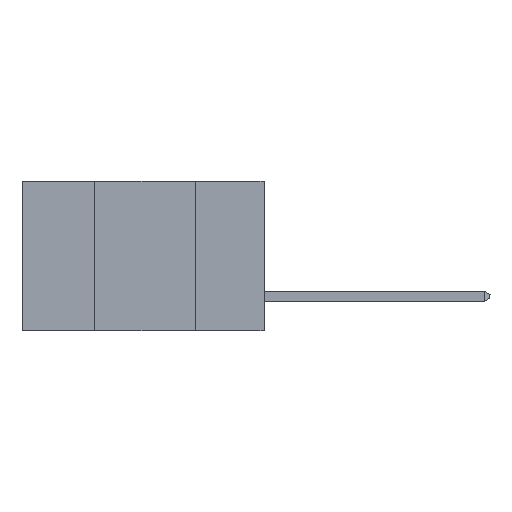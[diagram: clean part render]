
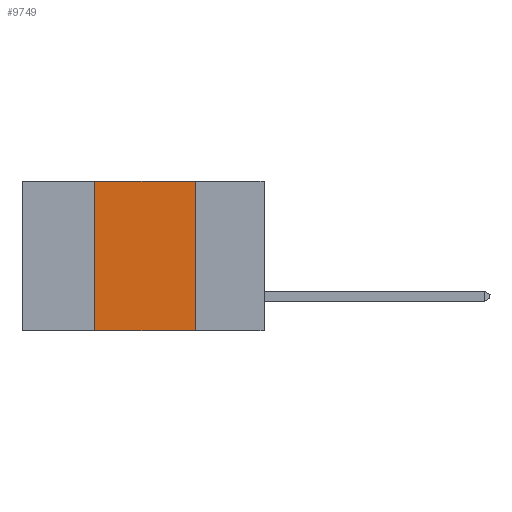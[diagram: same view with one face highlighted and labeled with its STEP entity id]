
A CAD part, left-side view. The second image highlights one B-rep face of the part: STEP entity #9749.
In plain terms, the highlighted planar face has unit normal (-1, 0, 0).
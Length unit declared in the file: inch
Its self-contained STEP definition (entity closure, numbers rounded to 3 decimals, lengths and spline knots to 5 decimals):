
#68 = VECTOR ( 'NONE', #13212, 39.37008 ) ;
#1419 = CARTESIAN_POINT ( 'NONE',  ( 0., 0.6, 0. ) ) ;
#1623 = CARTESIAN_POINT ( 'NONE',  ( 0., 0.6, 0. ) ) ;
#2707 = LINE ( 'NONE', #16694, #68 ) ;
#3376 = VECTOR ( 'NONE', #12726, 39.37008 ) ;
#3648 = CARTESIAN_POINT ( 'NONE',  ( 0., 0.42, 0. ) ) ;
#3920 = VERTEX_POINT ( 'NONE', #20898 ) ;
#5932 = DIRECTION ( 'NONE',  ( 0., 0., 1. ) ) ;
#6000 = CARTESIAN_POINT ( 'NONE',  ( 0., 0.42, 0. ) ) ;
#6022 = ORIENTED_EDGE ( 'NONE', *, *, #17591, .F. ) ;
#6243 = ORIENTED_EDGE ( 'NONE', *, *, #9950, .F. ) ;
#6796 = EDGE_LOOP ( 'NONE', ( #6243, #6022, #8694, #12789 ) ) ;
#7704 = EDGE_CURVE ( 'NONE', #11482, #11781, #21202, .T. ) ;
#8694 = ORIENTED_EDGE ( 'NONE', *, *, #21091, .F. ) ;
#9065 = CARTESIAN_POINT ( 'NONE',  ( 0., 0.6, -0.37 ) ) ;
#9735 = DIRECTION ( 'NONE',  ( 1., 0., 0. ) ) ;
#9749 = ADVANCED_FACE ( 'NONE', ( #12823 ), #19707, .F. ) ;
#9950 = EDGE_CURVE ( 'NONE', #3920, #11781, #2707, .T. ) ;
#10444 = CARTESIAN_POINT ( 'NONE',  ( 0., 0.17, -0.37 ) ) ;
#10857 = LINE ( 'NONE', #6000, #20985 ) ;
#11482 = VERTEX_POINT ( 'NONE', #17626 ) ;
#11617 = VERTEX_POINT ( 'NONE', #3648 ) ;
#11781 = VERTEX_POINT ( 'NONE', #10444 ) ;
#12192 = LINE ( 'NONE', #1419, #3376 ) ;
#12726 = DIRECTION ( 'NONE',  ( 0., -1., 0. ) ) ;
#12789 = ORIENTED_EDGE ( 'NONE', *, *, #7704, .T. ) ;
#12823 = FACE_OUTER_BOUND ( 'NONE', #6796, .T. ) ;
#13212 = DIRECTION ( 'NONE',  ( 0., 0., -1. ) ) ;
#13666 = AXIS2_PLACEMENT_3D ( 'NONE', #1623, #9735, #14632 ) ;
#14632 = DIRECTION ( 'NONE',  ( 0., 0., -1. ) ) ;
#15252 = VECTOR ( 'NONE', #17364, 39.37008 ) ;
#16694 = CARTESIAN_POINT ( 'NONE',  ( 0., 0.17, 0. ) ) ;
#17364 = DIRECTION ( 'NONE',  ( 0., -1., 0. ) ) ;
#17591 = EDGE_CURVE ( 'NONE', #11617, #3920, #12192, .T. ) ;
#17626 = CARTESIAN_POINT ( 'NONE',  ( 0., 0.42, -0.37 ) ) ;
#19707 = PLANE ( 'NONE',  #13666 ) ;
#20898 = CARTESIAN_POINT ( 'NONE',  ( 0., 0.17, 0. ) ) ;
#20985 = VECTOR ( 'NONE', #5932, 39.37008 ) ;
#21091 = EDGE_CURVE ( 'NONE', #11482, #11617, #10857, .T. ) ;
#21202 = LINE ( 'NONE', #9065, #15252 ) ;
